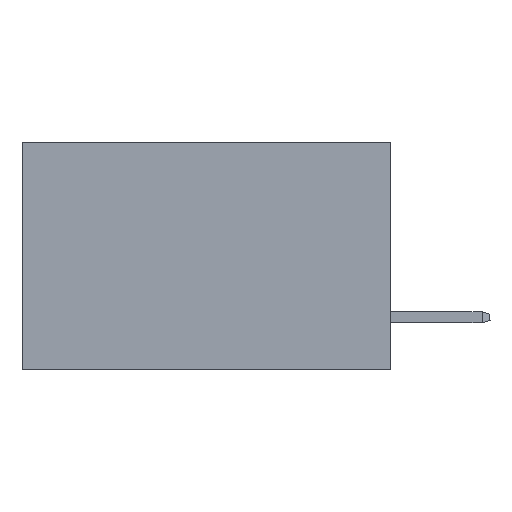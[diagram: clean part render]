
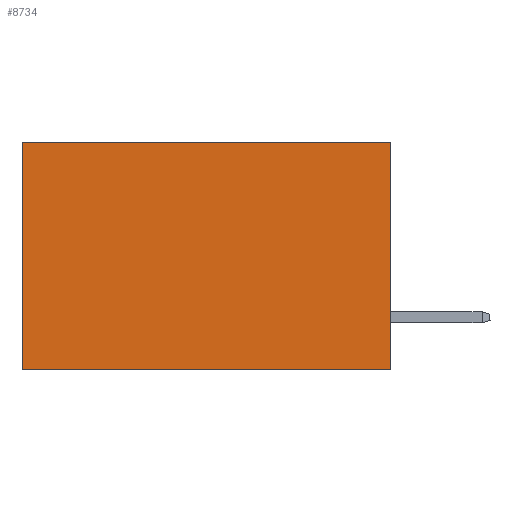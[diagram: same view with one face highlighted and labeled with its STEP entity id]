
A CAD part, left-side view. The second image highlights one B-rep face of the part: STEP entity #8734.
In plain terms, the highlighted planar face has unit normal (-1, 0, 0).
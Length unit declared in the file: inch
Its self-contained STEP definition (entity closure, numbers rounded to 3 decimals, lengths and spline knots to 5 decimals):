
#666 = EDGE_CURVE ( 'NONE', #38533, #39726, #1223, .T. ) ;
#1223 = LINE ( 'NONE', #18265, #25304 ) ;
#1770 = VECTOR ( 'NONE', #17030, 39.37008 ) ;
#1891 = AXIS2_PLACEMENT_3D ( 'NONE', #20928, #3836, #13848 ) ;
#2279 = ORIENTED_EDGE ( 'NONE', *, *, #666, .F. ) ;
#3836 = DIRECTION ( 'NONE',  ( 1., 0., 0. ) ) ;
#4466 = ORIENTED_EDGE ( 'NONE', *, *, #13737, .F. ) ;
#5308 = VERTEX_POINT ( 'NONE', #29472 ) ;
#7011 = EDGE_CURVE ( 'NONE', #5308, #23054, #21481, .T. ) ;
#8734 = ADVANCED_FACE ( 'NONE', ( #15921 ), #23787, .F. ) ;
#13737 = EDGE_CURVE ( 'NONE', #5308, #38533, #39682, .T. ) ;
#13842 = CARTESIAN_POINT ( 'NONE',  ( 0.2875, 0., 0. ) ) ;
#13848 = DIRECTION ( 'NONE',  ( 0., 0., -1. ) ) ;
#13854 = DIRECTION ( 'NONE',  ( 0., 0., -1. ) ) ;
#14045 = CARTESIAN_POINT ( 'NONE',  ( 0.2875, 0.6, -0.37 ) ) ;
#14532 = CARTESIAN_POINT ( 'NONE',  ( 0.2875, 0.6, 0. ) ) ;
#15921 = FACE_OUTER_BOUND ( 'NONE', #31216, .T. ) ;
#16772 = CARTESIAN_POINT ( 'NONE',  ( 0.2875, 0.6, 0. ) ) ;
#17030 = DIRECTION ( 'NONE',  ( 0., 1., 0. ) ) ;
#18265 = CARTESIAN_POINT ( 'NONE',  ( 0.2875, 0., -0.37 ) ) ;
#18924 = VECTOR ( 'NONE', #36576, 39.37008 ) ;
#19253 = EDGE_CURVE ( 'NONE', #23054, #39726, #32592, .T. ) ;
#19824 = CARTESIAN_POINT ( 'NONE',  ( 0.2875, 0., -0.37 ) ) ;
#20928 = CARTESIAN_POINT ( 'NONE',  ( 0.2875, 0., 0. ) ) ;
#21481 = LINE ( 'NONE', #13842, #1770 ) ;
#23054 = VERTEX_POINT ( 'NONE', #16772 ) ;
#23787 = PLANE ( 'NONE',  #1891 ) ;
#23816 = ORIENTED_EDGE ( 'NONE', *, *, #7011, .T. ) ;
#25304 = VECTOR ( 'NONE', #40361, 39.37008 ) ;
#29464 = CARTESIAN_POINT ( 'NONE',  ( 0.2875, 0., 0. ) ) ;
#29472 = CARTESIAN_POINT ( 'NONE',  ( 0.2875, 0., 0. ) ) ;
#31216 = EDGE_LOOP ( 'NONE', ( #36237, #2279, #4466, #23816 ) ) ;
#31292 = VECTOR ( 'NONE', #13854, 39.37008 ) ;
#32592 = LINE ( 'NONE', #14532, #18924 ) ;
#36237 = ORIENTED_EDGE ( 'NONE', *, *, #19253, .T. ) ;
#36576 = DIRECTION ( 'NONE',  ( 0., 0., -1. ) ) ;
#38533 = VERTEX_POINT ( 'NONE', #19824 ) ;
#39682 = LINE ( 'NONE', #29464, #31292 ) ;
#39726 = VERTEX_POINT ( 'NONE', #14045 ) ;
#40361 = DIRECTION ( 'NONE',  ( 0., 1., 0. ) ) ;
